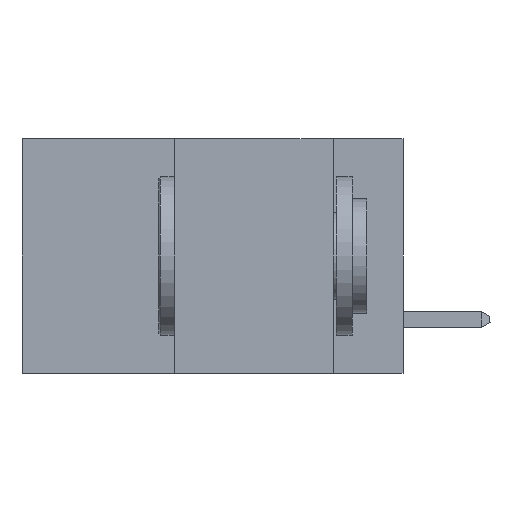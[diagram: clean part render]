
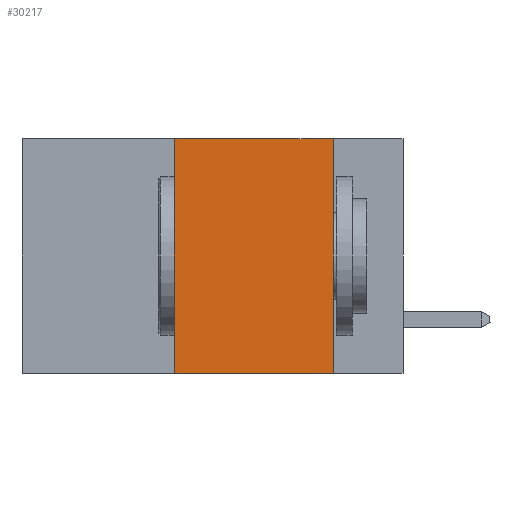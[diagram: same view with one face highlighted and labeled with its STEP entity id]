
A CAD part, left-side view. The second image highlights one B-rep face of the part: STEP entity #30217.
In plain terms, the highlighted planar face has unit normal (-1, 0, 0).
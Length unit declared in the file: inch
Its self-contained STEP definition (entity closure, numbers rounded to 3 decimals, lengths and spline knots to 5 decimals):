
#57 = DIRECTION ( 'NONE',  ( 0., 0., -1. ) ) ;
#442 = VERTEX_POINT ( 'NONE', #45466 ) ;
#7009 = VERTEX_POINT ( 'NONE', #10256 ) ;
#10034 = EDGE_CURVE ( 'NONE', #442, #30245, #45580, .T. ) ;
#10256 = CARTESIAN_POINT ( 'NONE',  ( 0., 0.11, 0. ) ) ;
#10891 = ORIENTED_EDGE ( 'NONE', *, *, #34011, .F. ) ;
#10903 = AXIS2_PLACEMENT_3D ( 'NONE', #38161, #44514, #57 ) ;
#12085 = EDGE_LOOP ( 'NONE', ( #42423, #25999, #10891, #43746 ) ) ;
#12139 = CARTESIAN_POINT ( 'NONE',  ( 0., 0.36, 0. ) ) ;
#12911 = DIRECTION ( 'NONE',  ( 0., 0., -1. ) ) ;
#22429 = VECTOR ( 'NONE', #40066, 39.37008 ) ;
#23120 = CARTESIAN_POINT ( 'NONE',  ( 0., 0.11, -0.37 ) ) ;
#23297 = LINE ( 'NONE', #12139, #27440 ) ;
#25999 = ORIENTED_EDGE ( 'NONE', *, *, #30783, .F. ) ;
#27440 = VECTOR ( 'NONE', #38610, 39.37008 ) ;
#30217 = ADVANCED_FACE ( 'NONE', ( #47398 ), #36846, .F. ) ;
#30245 = VERTEX_POINT ( 'NONE', #23120 ) ;
#30783 = EDGE_CURVE ( 'NONE', #42933, #7009, #44329, .T. ) ;
#31386 = LINE ( 'NONE', #46267, #35537 ) ;
#33912 = CARTESIAN_POINT ( 'NONE',  ( 0., 0.6, 0. ) ) ;
#34011 = EDGE_CURVE ( 'NONE', #442, #42933, #23297, .T. ) ;
#35537 = VECTOR ( 'NONE', #12911, 39.37008 ) ;
#36596 = VECTOR ( 'NONE', #45420, 39.37008 ) ;
#36846 = PLANE ( 'NONE',  #10903 ) ;
#36890 = CARTESIAN_POINT ( 'NONE',  ( 0., 0.36, 0. ) ) ;
#38161 = CARTESIAN_POINT ( 'NONE',  ( 0., 0.6, 0. ) ) ;
#38610 = DIRECTION ( 'NONE',  ( 0., 0., 1. ) ) ;
#39903 = CARTESIAN_POINT ( 'NONE',  ( 0., 0.6, -0.37 ) ) ;
#40066 = DIRECTION ( 'NONE',  ( 0., -1., 0. ) ) ;
#42423 = ORIENTED_EDGE ( 'NONE', *, *, #48391, .F. ) ;
#42933 = VERTEX_POINT ( 'NONE', #36890 ) ;
#43746 = ORIENTED_EDGE ( 'NONE', *, *, #10034, .T. ) ;
#44329 = LINE ( 'NONE', #33912, #36596 ) ;
#44514 = DIRECTION ( 'NONE',  ( 1., 0., 0. ) ) ;
#45420 = DIRECTION ( 'NONE',  ( 0., -1., 0. ) ) ;
#45466 = CARTESIAN_POINT ( 'NONE',  ( 0., 0.36, -0.37 ) ) ;
#45580 = LINE ( 'NONE', #39903, #22429 ) ;
#46267 = CARTESIAN_POINT ( 'NONE',  ( 0., 0.11, 0. ) ) ;
#47398 = FACE_OUTER_BOUND ( 'NONE', #12085, .T. ) ;
#48391 = EDGE_CURVE ( 'NONE', #7009, #30245, #31386, .T. ) ;
